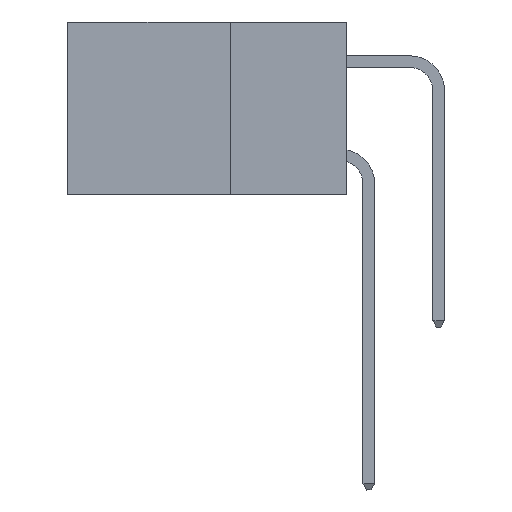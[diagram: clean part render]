
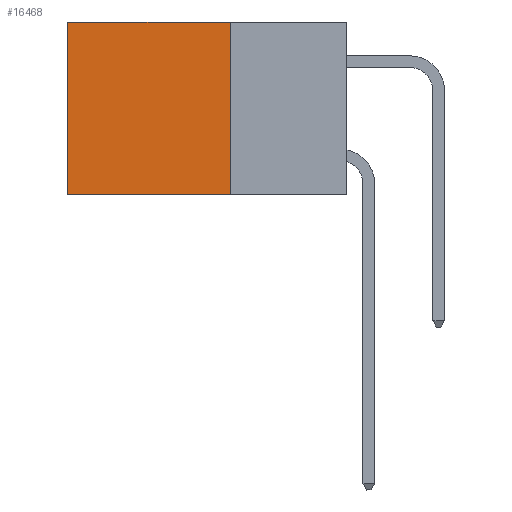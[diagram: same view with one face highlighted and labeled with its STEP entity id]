
A CAD part, left-side view. The second image highlights one B-rep face of the part: STEP entity #16468.
In plain terms, the highlighted planar face has unit normal (-1, 0, 0).
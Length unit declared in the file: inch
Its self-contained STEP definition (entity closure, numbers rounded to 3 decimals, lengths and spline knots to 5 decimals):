
#480 = VERTEX_POINT ( 'NONE', #6180 ) ;
#665 = ORIENTED_EDGE ( 'NONE', *, *, #13470, .T. ) ;
#830 = VECTOR ( 'NONE', #5380, 39.37008 ) ;
#1125 = AXIS2_PLACEMENT_3D ( 'NONE', #17768, #6906, #4063 ) ;
#1198 = EDGE_CURVE ( 'NONE', #9096, #480, #12237, .T. ) ;
#1454 = DIRECTION ( 'NONE',  ( 0., 0., -1. ) ) ;
#1683 = CARTESIAN_POINT ( 'NONE',  ( 0.2875, 0.25, -0.37 ) ) ;
#3680 = CARTESIAN_POINT ( 'NONE',  ( 0.2875, 0.25, 0. ) ) ;
#3812 = VERTEX_POINT ( 'NONE', #4949 ) ;
#4063 = DIRECTION ( 'NONE',  ( 0., 0., -1. ) ) ;
#4949 = CARTESIAN_POINT ( 'NONE',  ( 0.2875, 0.6, -0.37 ) ) ;
#5380 = DIRECTION ( 'NONE',  ( 0., 0., -1. ) ) ;
#6180 = CARTESIAN_POINT ( 'NONE',  ( 0.2875, 0.6, 0. ) ) ;
#6906 = DIRECTION ( 'NONE',  ( 1., 0., 0. ) ) ;
#8670 = CARTESIAN_POINT ( 'NONE',  ( 0.2875, 0.25, 0. ) ) ;
#8806 = LINE ( 'NONE', #1683, #11762 ) ;
#9091 = DIRECTION ( 'NONE',  ( 0., 1., 0. ) ) ;
#9096 = VERTEX_POINT ( 'NONE', #13260 ) ;
#9231 = CARTESIAN_POINT ( 'NONE',  ( 0.2875, 0.25, -0.37 ) ) ;
#11614 = LINE ( 'NONE', #8670, #13840 ) ;
#11762 = VECTOR ( 'NONE', #9091, 39.37008 ) ;
#11943 = PLANE ( 'NONE',  #1125 ) ;
#12237 = LINE ( 'NONE', #3680, #16918 ) ;
#13260 = CARTESIAN_POINT ( 'NONE',  ( 0.2875, 0.25, 0. ) ) ;
#13380 = FACE_OUTER_BOUND ( 'NONE', #18781, .T. ) ;
#13470 = EDGE_CURVE ( 'NONE', #480, #3812, #18795, .T. ) ;
#13840 = VECTOR ( 'NONE', #1454, 39.37008 ) ;
#14181 = VERTEX_POINT ( 'NONE', #9231 ) ;
#14799 = ORIENTED_EDGE ( 'NONE', *, *, #15385, .F. ) ;
#14967 = ORIENTED_EDGE ( 'NONE', *, *, #17744, .F. ) ;
#15281 = DIRECTION ( 'NONE',  ( 0., 1., 0. ) ) ;
#15385 = EDGE_CURVE ( 'NONE', #9096, #14181, #11614, .T. ) ;
#15997 = ORIENTED_EDGE ( 'NONE', *, *, #1198, .T. ) ;
#16468 = ADVANCED_FACE ( 'NONE', ( #13380 ), #11943, .F. ) ;
#16918 = VECTOR ( 'NONE', #15281, 39.37008 ) ;
#17744 = EDGE_CURVE ( 'NONE', #14181, #3812, #8806, .T. ) ;
#17768 = CARTESIAN_POINT ( 'NONE',  ( 0.2875, 0.25, 0. ) ) ;
#18430 = CARTESIAN_POINT ( 'NONE',  ( 0.2875, 0.6, 0. ) ) ;
#18781 = EDGE_LOOP ( 'NONE', ( #665, #14967, #14799, #15997 ) ) ;
#18795 = LINE ( 'NONE', #18430, #830 ) ;
